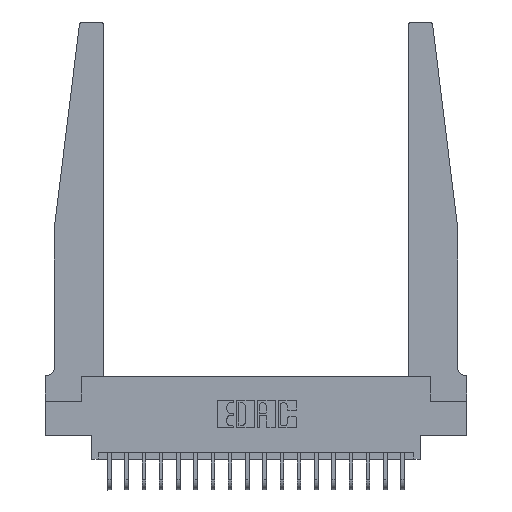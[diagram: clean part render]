
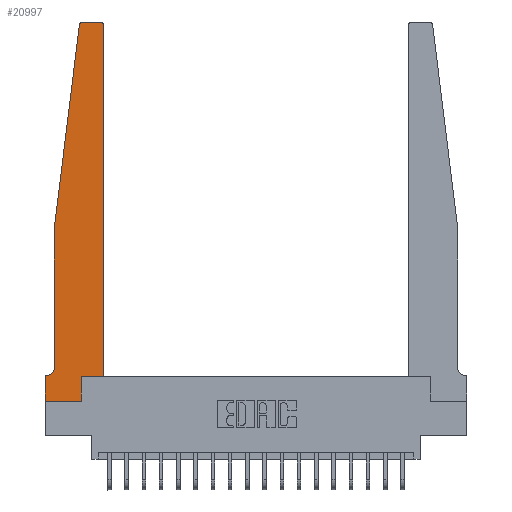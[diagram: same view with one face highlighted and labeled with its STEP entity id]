
A CAD part, top view. The second image highlights one B-rep face of the part: STEP entity #20997.
In plain terms, the highlighted planar face has unit normal (0, 0, 1).
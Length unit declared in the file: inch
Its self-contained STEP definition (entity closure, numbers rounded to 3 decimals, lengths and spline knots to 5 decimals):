
#68 = CARTESIAN_POINT ( 'NONE',  ( 0.425, 0.18, 0.37 ) ) ;
#436 = DIRECTION ( 'NONE',  ( -1., 0., 0. ) ) ;
#459 = CARTESIAN_POINT ( 'NONE',  ( 0.065, 1.25, 0.37 ) ) ;
#637 = LINE ( 'NONE', #12689, #14583 ) ;
#798 = EDGE_LOOP ( 'NONE', ( #13687, #5420, #1403, #13355, #17013, #8809, #19973, #2349, #3820, #21486, #6416, #1933 ) ) ;
#1250 = CARTESIAN_POINT ( 'NONE',  ( 0.395, 2.72, 0.37 ) ) ;
#1283 = CIRCLE ( 'NONE', #15263, 0.03 ) ;
#1300 = EDGE_CURVE ( 'NONE', #2958, #21305, #21213, .T. ) ;
#1403 = ORIENTED_EDGE ( 'NONE', *, *, #20076, .T. ) ;
#1933 = ORIENTED_EDGE ( 'NONE', *, *, #9886, .T. ) ;
#2349 = ORIENTED_EDGE ( 'NONE', *, *, #6894, .T. ) ;
#2519 = VECTOR ( 'NONE', #3661, 39.37008 ) ;
#2898 = CARTESIAN_POINT ( 'NONE',  ( 0.065, 1.25, 0.37 ) ) ;
#2958 = VERTEX_POINT ( 'NONE', #459 ) ;
#3041 = VECTOR ( 'NONE', #436, 39.37008 ) ;
#3211 = DIRECTION ( 'NONE',  ( 0., 0., 1. ) ) ;
#3410 = VECTOR ( 'NONE', #7363, 39.37008 ) ;
#3465 = EDGE_CURVE ( 'NONE', #8928, #6980, #6999, .T. ) ;
#3661 = DIRECTION ( 'NONE',  ( 0., 1., 0. ) ) ;
#3666 = EDGE_CURVE ( 'NONE', #21305, #16962, #16691, .T. ) ;
#3755 = CARTESIAN_POINT ( 'NONE',  ( 0.425, 0.18, 0.37 ) ) ;
#3820 = ORIENTED_EDGE ( 'NONE', *, *, #12730, .T. ) ;
#4162 = AXIS2_PLACEMENT_3D ( 'NONE', #15392, #16957, #20322 ) ;
#4489 = DIRECTION ( 'NONE',  ( 0., 1., 0. ) ) ;
#4784 = CARTESIAN_POINT ( 'NONE',  ( 0.25, 2.75, 0.37 ) ) ;
#4920 = CARTESIAN_POINT ( 'NONE',  ( 0.24675, 2.72367, 0.37 ) ) ;
#5010 = VECTOR ( 'NONE', #12796, 39.37008 ) ;
#5026 = VERTEX_POINT ( 'NONE', #14857 ) ;
#5420 = ORIENTED_EDGE ( 'NONE', *, *, #21590, .T. ) ;
#5645 = CARTESIAN_POINT ( 'NONE',  ( 0.015, 0.2375, 0.37 ) ) ;
#5788 = DIRECTION ( 'NONE',  ( -1., 0., 0. ) ) ;
#6321 = DIRECTION ( 'NONE',  ( 1., 0., 0. ) ) ;
#6416 = ORIENTED_EDGE ( 'NONE', *, *, #11421, .T. ) ;
#6754 = CARTESIAN_POINT ( 'NONE',  ( 0.27653, 2.75, 0.37 ) ) ;
#6894 = EDGE_CURVE ( 'NONE', #20549, #11818, #20744, .T. ) ;
#6980 = VERTEX_POINT ( 'NONE', #6754 ) ;
#6999 = LINE ( 'NONE', #4784, #3041 ) ;
#7286 = DIRECTION ( 'NONE',  ( 1., 0., 0. ) ) ;
#7362 = CARTESIAN_POINT ( 'NONE',  ( 0.015, 0.1875, 0.37 ) ) ;
#7363 = DIRECTION ( 'NONE',  ( 0., -1., 0. ) ) ;
#7537 = AXIS2_PLACEMENT_3D ( 'NONE', #14000, #20764, #14074 ) ;
#7829 = DIRECTION ( 'NONE',  ( -0.122, -0.992, 0. ) ) ;
#7900 = EDGE_CURVE ( 'NONE', #16962, #19462, #9684, .T. ) ;
#7965 = CARTESIAN_POINT ( 'NONE',  ( 0.065, 0.2375, 0.37 ) ) ;
#8115 = CARTESIAN_POINT ( 'NONE',  ( 0., 0., 0.37 ) ) ;
#8168 = EDGE_CURVE ( 'NONE', #17344, #5026, #8406, .T. ) ;
#8406 = LINE ( 'NONE', #3755, #13942 ) ;
#8809 = ORIENTED_EDGE ( 'NONE', *, *, #7900, .T. ) ;
#8928 = VERTEX_POINT ( 'NONE', #15041 ) ;
#9486 = EDGE_CURVE ( 'NONE', #19462, #20549, #9667, .T. ) ;
#9667 = LINE ( 'NONE', #17167, #10714 ) ;
#9684 = LINE ( 'NONE', #11238, #5010 ) ;
#9842 = LINE ( 'NONE', #68, #2519 ) ;
#9859 = VERTEX_POINT ( 'NONE', #4920 ) ;
#9886 = EDGE_CURVE ( 'NONE', #11595, #8928, #1283, .T. ) ;
#9978 = LINE ( 'NONE', #2898, #20219 ) ;
#10714 = VECTOR ( 'NONE', #20384, 39.37008 ) ;
#11238 = CARTESIAN_POINT ( 'NONE',  ( 0.065, 0.1875, 0.37 ) ) ;
#11421 = EDGE_CURVE ( 'NONE', #5026, #11595, #9842, .T. ) ;
#11595 = VERTEX_POINT ( 'NONE', #20913 ) ;
#11818 = VERTEX_POINT ( 'NONE', #12955 ) ;
#11896 = DIRECTION ( 'NONE',  ( 1., 0., 0. ) ) ;
#12163 = FACE_OUTER_BOUND ( 'NONE', #798, .T. ) ;
#12689 = CARTESIAN_POINT ( 'NONE',  ( 0.2605, 0.18, 0.37 ) ) ;
#12730 = EDGE_CURVE ( 'NONE', #11818, #17344, #637, .T. ) ;
#12796 = DIRECTION ( 'NONE',  ( -1., 0., 0. ) ) ;
#12955 = CARTESIAN_POINT ( 'NONE',  ( 0.2605, 0., 0.37 ) ) ;
#13355 = ORIENTED_EDGE ( 'NONE', *, *, #1300, .T. ) ;
#13687 = ORIENTED_EDGE ( 'NONE', *, *, #3465, .T. ) ;
#13745 = CIRCLE ( 'NONE', #4162, 0.03 ) ;
#13942 = VECTOR ( 'NONE', #11896, 39.37008 ) ;
#14000 = CARTESIAN_POINT ( 'NONE',  ( 0., 0.1875, 0.37 ) ) ;
#14074 = DIRECTION ( 'NONE',  ( 1., 0., 0. ) ) ;
#14583 = VECTOR ( 'NONE', #4489, 39.37008 ) ;
#14857 = CARTESIAN_POINT ( 'NONE',  ( 0.425, 0.18, 0.37 ) ) ;
#15041 = CARTESIAN_POINT ( 'NONE',  ( 0.395, 2.75, 0.37 ) ) ;
#15263 = AXIS2_PLACEMENT_3D ( 'NONE', #1250, #3211, #6321 ) ;
#15392 = CARTESIAN_POINT ( 'NONE',  ( 0.27653, 2.72, 0.37 ) ) ;
#15944 = CARTESIAN_POINT ( 'NONE',  ( 0.065, 1.25, 0.37 ) ) ;
#16691 = CIRCLE ( 'NONE', #17500, 0.05 ) ;
#16957 = DIRECTION ( 'NONE',  ( 0., 0., 1. ) ) ;
#16962 = VERTEX_POINT ( 'NONE', #7362 ) ;
#17013 = ORIENTED_EDGE ( 'NONE', *, *, #3666, .T. ) ;
#17167 = CARTESIAN_POINT ( 'NONE',  ( 0., 0., 0.37 ) ) ;
#17344 = VERTEX_POINT ( 'NONE', #20877 ) ;
#17356 = VECTOR ( 'NONE', #7286, 39.37008 ) ;
#17500 = AXIS2_PLACEMENT_3D ( 'NONE', #5645, #18955, #5788 ) ;
#17739 = CARTESIAN_POINT ( 'NONE',  ( 0., 0., 0.37 ) ) ;
#18085 = CARTESIAN_POINT ( 'NONE',  ( 0., 0.1875, 0.37 ) ) ;
#18955 = DIRECTION ( 'NONE',  ( 0., 0., -1. ) ) ;
#19147 = PLANE ( 'NONE',  #7537 ) ;
#19462 = VERTEX_POINT ( 'NONE', #18085 ) ;
#19973 = ORIENTED_EDGE ( 'NONE', *, *, #9486, .T. ) ;
#20076 = EDGE_CURVE ( 'NONE', #9859, #2958, #9978, .T. ) ;
#20219 = VECTOR ( 'NONE', #7829, 39.37008 ) ;
#20322 = DIRECTION ( 'NONE',  ( 1., 0., 0. ) ) ;
#20384 = DIRECTION ( 'NONE',  ( 0., -1., 0. ) ) ;
#20549 = VERTEX_POINT ( 'NONE', #17739 ) ;
#20744 = LINE ( 'NONE', #8115, #17356 ) ;
#20764 = DIRECTION ( 'NONE',  ( 0., 0., 1. ) ) ;
#20877 = CARTESIAN_POINT ( 'NONE',  ( 0.2605, 0.18, 0.37 ) ) ;
#20913 = CARTESIAN_POINT ( 'NONE',  ( 0.425, 2.72, 0.37 ) ) ;
#20997 = ADVANCED_FACE ( 'NONE', ( #12163 ), #19147, .T. ) ;
#21213 = LINE ( 'NONE', #15944, #3410 ) ;
#21305 = VERTEX_POINT ( 'NONE', #7965 ) ;
#21486 = ORIENTED_EDGE ( 'NONE', *, *, #8168, .T. ) ;
#21590 = EDGE_CURVE ( 'NONE', #6980, #9859, #13745, .T. ) ;
